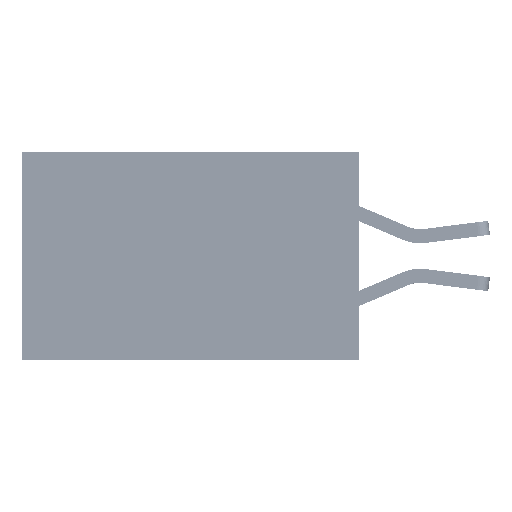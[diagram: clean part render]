
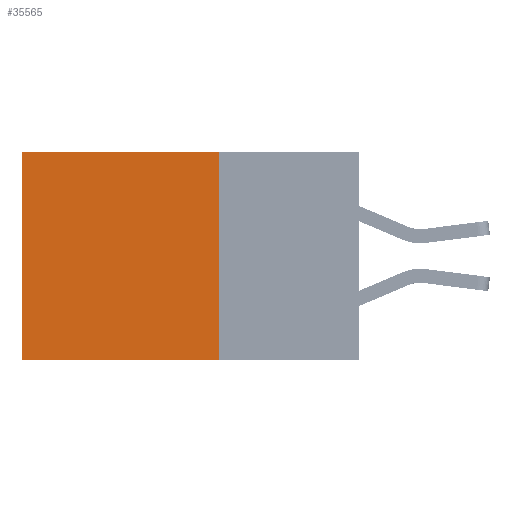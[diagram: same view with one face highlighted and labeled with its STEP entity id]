
A CAD part, left-side view. The second image highlights one B-rep face of the part: STEP entity #35565.
In plain terms, the highlighted planar face has unit normal (-1, 0, 0).
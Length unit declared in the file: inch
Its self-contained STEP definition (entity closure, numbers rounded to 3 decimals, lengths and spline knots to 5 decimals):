
#1985 = ORIENTED_EDGE ( 'NONE', *, *, #6692, .T. ) ;
#4240 = DIRECTION ( 'NONE',  ( 0., 0., -1. ) ) ;
#6518 = CARTESIAN_POINT ( 'NONE',  ( 0.2875, 0.25, 0. ) ) ;
#6692 = EDGE_CURVE ( 'NONE', #33961, #12530, #20805, .T. ) ;
#7635 = LINE ( 'NONE', #36691, #37727 ) ;
#7781 = FACE_OUTER_BOUND ( 'NONE', #23967, .T. ) ;
#10798 = CARTESIAN_POINT ( 'NONE',  ( 0.2875, 0.6, -0.37 ) ) ;
#11350 = PLANE ( 'NONE',  #22751 ) ;
#12530 = VERTEX_POINT ( 'NONE', #10798 ) ;
#12979 = VECTOR ( 'NONE', #4240, 39.37008 ) ;
#14308 = DIRECTION ( 'NONE',  ( 0., 0., -1. ) ) ;
#14444 = ORIENTED_EDGE ( 'NONE', *, *, #37296, .T. ) ;
#14445 = DIRECTION ( 'NONE',  ( 0., 0., -1. ) ) ;
#16736 = ORIENTED_EDGE ( 'NONE', *, *, #24770, .F. ) ;
#19786 = VERTEX_POINT ( 'NONE', #6518 ) ;
#20102 = CARTESIAN_POINT ( 'NONE',  ( 0.2875, 0.25, 0. ) ) ;
#20805 = LINE ( 'NONE', #36265, #12979 ) ;
#22570 = CARTESIAN_POINT ( 'NONE',  ( 0.2875, 0.25, -0.37 ) ) ;
#22751 = AXIS2_PLACEMENT_3D ( 'NONE', #20102, #31818, #14308 ) ;
#23180 = CARTESIAN_POINT ( 'NONE',  ( 0.2875, 0.25, 0. ) ) ;
#23519 = VERTEX_POINT ( 'NONE', #25842 ) ;
#23967 = EDGE_LOOP ( 'NONE', ( #1985, #16736, #29500, #14444 ) ) ;
#24389 = VECTOR ( 'NONE', #36962, 39.37008 ) ;
#24770 = EDGE_CURVE ( 'NONE', #23519, #12530, #32096, .T. ) ;
#25842 = CARTESIAN_POINT ( 'NONE',  ( 0.2875, 0.25, -0.37 ) ) ;
#27819 = VECTOR ( 'NONE', #14445, 39.37008 ) ;
#28418 = DIRECTION ( 'NONE',  ( 0., 1., 0. ) ) ;
#29500 = ORIENTED_EDGE ( 'NONE', *, *, #31747, .F. ) ;
#31747 = EDGE_CURVE ( 'NONE', #19786, #23519, #35460, .T. ) ;
#31818 = DIRECTION ( 'NONE',  ( 1., 0., 0. ) ) ;
#32096 = LINE ( 'NONE', #22570, #24389 ) ;
#33961 = VERTEX_POINT ( 'NONE', #37813 ) ;
#35460 = LINE ( 'NONE', #23180, #27819 ) ;
#35565 = ADVANCED_FACE ( 'NONE', ( #7781 ), #11350, .F. ) ;
#36265 = CARTESIAN_POINT ( 'NONE',  ( 0.2875, 0.6, 0. ) ) ;
#36691 = CARTESIAN_POINT ( 'NONE',  ( 0.2875, 0.25, 0. ) ) ;
#36962 = DIRECTION ( 'NONE',  ( 0., 1., 0. ) ) ;
#37296 = EDGE_CURVE ( 'NONE', #19786, #33961, #7635, .T. ) ;
#37727 = VECTOR ( 'NONE', #28418, 39.37008 ) ;
#37813 = CARTESIAN_POINT ( 'NONE',  ( 0.2875, 0.6, 0. ) ) ;
